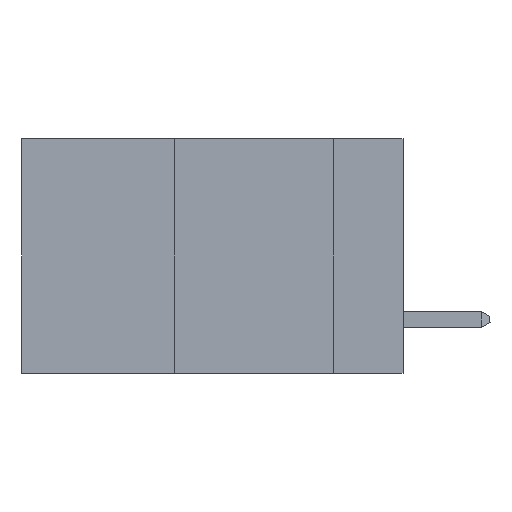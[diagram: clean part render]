
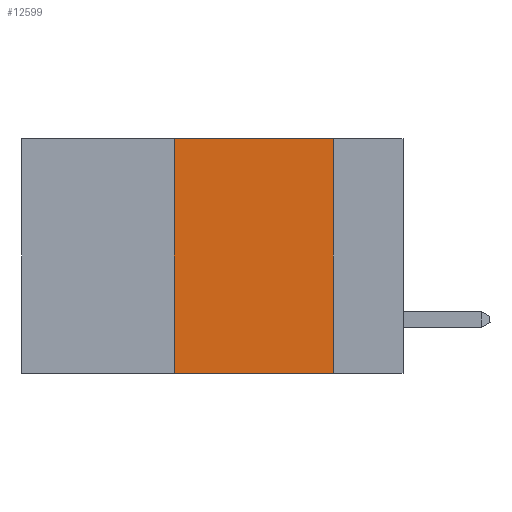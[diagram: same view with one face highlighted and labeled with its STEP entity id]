
A CAD part, left-side view. The second image highlights one B-rep face of the part: STEP entity #12599.
In plain terms, the highlighted planar face has unit normal (-1, 0, 0).
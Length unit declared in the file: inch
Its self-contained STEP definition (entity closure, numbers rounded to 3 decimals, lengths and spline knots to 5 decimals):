
#1005 = CARTESIAN_POINT ( 'NONE',  ( 0., 0.6, 0. ) ) ;
#1053 = CARTESIAN_POINT ( 'NONE',  ( 0., 0.6, -0.37 ) ) ;
#1134 = LINE ( 'NONE', #12970, #2439 ) ;
#1245 = AXIS2_PLACEMENT_3D ( 'NONE', #6454, #8474, #12869 ) ;
#1461 = ORIENTED_EDGE ( 'NONE', *, *, #6795, .F. ) ;
#1639 = LINE ( 'NONE', #1053, #12679 ) ;
#1850 = EDGE_CURVE ( 'NONE', #10237, #6545, #6261, .T. ) ;
#1903 = ORIENTED_EDGE ( 'NONE', *, *, #5611, .F. ) ;
#1939 = VECTOR ( 'NONE', #2678, 39.37008 ) ;
#2122 = DIRECTION ( 'NONE',  ( 0., -1., 0. ) ) ;
#2439 = VECTOR ( 'NONE', #11727, 39.37008 ) ;
#2678 = DIRECTION ( 'NONE',  ( 0., 0., -1. ) ) ;
#2704 = CARTESIAN_POINT ( 'NONE',  ( 0., 0.11, -0.37 ) ) ;
#2968 = FACE_OUTER_BOUND ( 'NONE', #5109, .T. ) ;
#4710 = VECTOR ( 'NONE', #8421, 39.37008 ) ;
#4723 = LINE ( 'NONE', #12207, #1939 ) ;
#5109 = EDGE_LOOP ( 'NONE', ( #1461, #8360, #1903, #5286 ) ) ;
#5286 = ORIENTED_EDGE ( 'NONE', *, *, #12668, .T. ) ;
#5611 = EDGE_CURVE ( 'NONE', #7159, #10237, #1134, .T. ) ;
#6261 = LINE ( 'NONE', #1005, #4710 ) ;
#6454 = CARTESIAN_POINT ( 'NONE',  ( 0., 0.6, 0. ) ) ;
#6545 = VERTEX_POINT ( 'NONE', #8149 ) ;
#6795 = EDGE_CURVE ( 'NONE', #6545, #7455, #4723, .T. ) ;
#7159 = VERTEX_POINT ( 'NONE', #12648 ) ;
#7455 = VERTEX_POINT ( 'NONE', #2704 ) ;
#8149 = CARTESIAN_POINT ( 'NONE',  ( 0., 0.11, 0. ) ) ;
#8360 = ORIENTED_EDGE ( 'NONE', *, *, #1850, .F. ) ;
#8421 = DIRECTION ( 'NONE',  ( 0., -1., 0. ) ) ;
#8474 = DIRECTION ( 'NONE',  ( 1., 0., 0. ) ) ;
#8607 = PLANE ( 'NONE',  #1245 ) ;
#10237 = VERTEX_POINT ( 'NONE', #11170 ) ;
#11170 = CARTESIAN_POINT ( 'NONE',  ( 0., 0.36, 0. ) ) ;
#11727 = DIRECTION ( 'NONE',  ( 0., 0., 1. ) ) ;
#12207 = CARTESIAN_POINT ( 'NONE',  ( 0., 0.11, 0. ) ) ;
#12599 = ADVANCED_FACE ( 'NONE', ( #2968 ), #8607, .F. ) ;
#12648 = CARTESIAN_POINT ( 'NONE',  ( 0., 0.36, -0.37 ) ) ;
#12668 = EDGE_CURVE ( 'NONE', #7159, #7455, #1639, .T. ) ;
#12679 = VECTOR ( 'NONE', #2122, 39.37008 ) ;
#12869 = DIRECTION ( 'NONE',  ( 0., 0., -1. ) ) ;
#12970 = CARTESIAN_POINT ( 'NONE',  ( 0., 0.36, 0. ) ) ;
